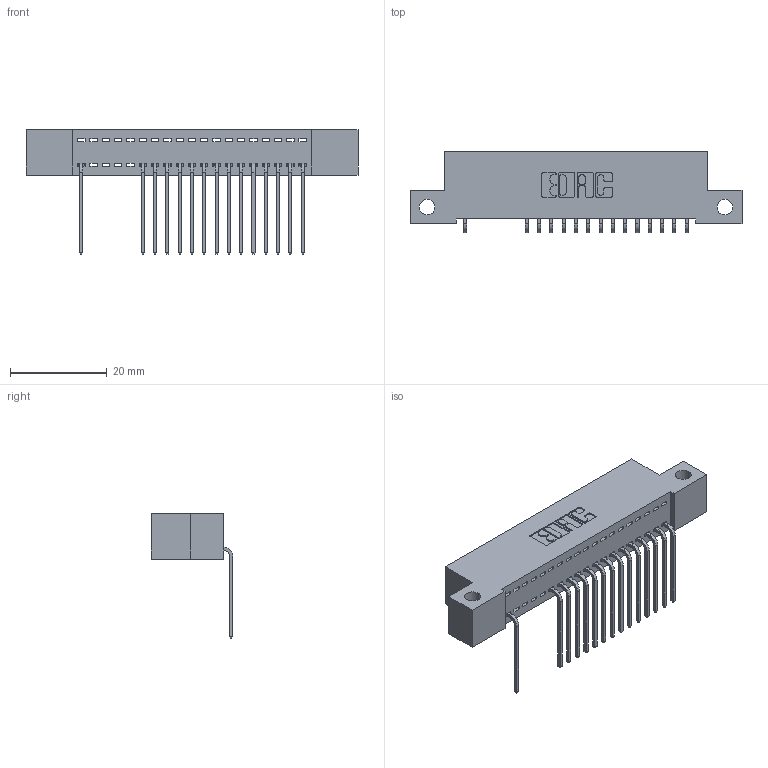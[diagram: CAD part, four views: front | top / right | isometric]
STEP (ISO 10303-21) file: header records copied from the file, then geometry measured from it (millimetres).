
FILE_DESCRIPTION (( 'STEP AP203' ), '1' );
FILE_NAME ('392-019-559-112.STEP', '2018-08-15T05:48:40', ( '' ), ( '' ), 'SwSTEP 2.0', 'SolidWorks 2016', '' );
FILE_SCHEMA (( 'CONFIG_CONTROL_DESIGN' ));
Length unit declared in the file: inch
Products named in the file (3): 392-019-559-112; 342 Part_Side Mount; 345-292-001_558 559 Tail - 1
Assembly tree (16 placements, depth 2):
  392-019-559-112
    342 Part_Side Mount
    345-292-001_558 559 Tail - 1  x15
Bounding box: 68.58 x 16.83 x 25.78 mm (x, y, z)
Volume: 5858.7 mm3; surface area: 8057.5 mm2
Topology: 16 solids, 16 shells, 1058 faces, 3197 edges, 2110 vertices
Faces by surface type: plane 774, cylinder 284
Entity records: 14417 total; most frequent: CARTESIAN_POINT 2515, ORIENTED_EDGE 2474, DIRECTION 2163, EDGE_CURVE 1237, VECTOR 1109, LINE 1109, VERTEX_POINT 822, AXIS2_PLACEMENT_3D 527
